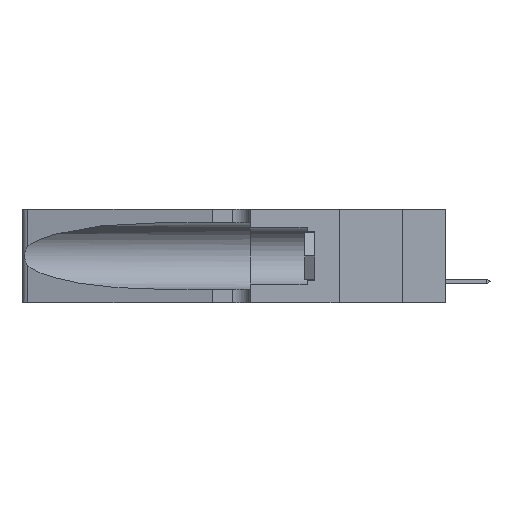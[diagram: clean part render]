
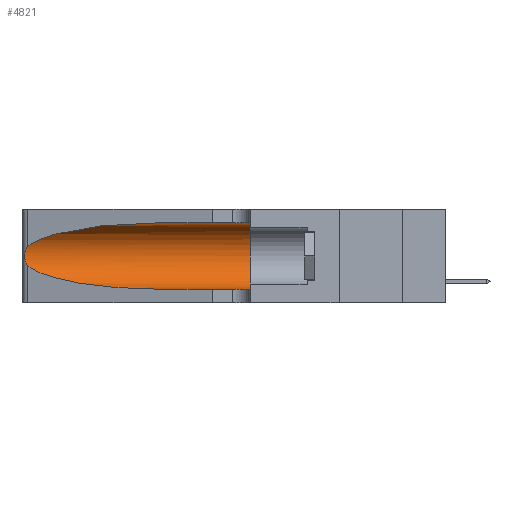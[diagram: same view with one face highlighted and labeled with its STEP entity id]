
A CAD part, left-side view. The second image highlights one B-rep face of the part: STEP entity #4821.
In plain terms, the highlighted cylindrical face has radius 3.308 mm (diameter 6.617 mm), a partial arc.
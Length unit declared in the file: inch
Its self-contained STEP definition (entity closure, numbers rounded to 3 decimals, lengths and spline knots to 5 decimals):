
#594 = B_SPLINE_CURVE_WITH_KNOTS ( 'NONE', 3,
 ( #18138, #36412, #43716, #26336, #4573, #8216, #18551, #36834, #26012, #4256, #18857, #44283, #20702, #31666 ),
 .UNSPECIFIED., .F., .F.,
 ( 4, 2, 2, 2, 2, 2, 4 ),
 ( 0., 0.00027, 0.00053, 0.00107, 0.0016, 0.00187, 0.00214 ),
 .UNSPECIFIED. ) ;
#1553 = DIRECTION ( 'NONE',  ( 0., -1., 0. ) ) ;
#2126 = EDGE_CURVE ( 'NONE', #46889, #8307, #594, .T. ) ;
#2876 = ORIENTED_EDGE ( 'NONE', *, *, #18980, .F. ) ;
#3038 = ORIENTED_EDGE ( 'NONE', *, *, #10313, .T. ) ;
#4256 = CARTESIAN_POINT ( 'NONE',  ( 0.25856, 1.23593, 0.16098 ) ) ;
#4573 = CARTESIAN_POINT ( 'NONE',  ( 0.25854, 1.2359, 0.20912 ) ) ;
#4821 = ADVANCED_FACE ( 'NONE', ( #39656 ), #5519, .F. ) ;
#4877 = VERTEX_POINT ( 'NONE', #45005 ) ;
#5519 = CYLINDRICAL_SURFACE ( 'NONE', #36890, 0.13025 ) ;
#7136 = CARTESIAN_POINT ( 'NONE',  ( 0.25487, 1.22718, 0.22369 ) ) ;
#8213 = CARTESIAN_POINT ( 'NONE',  ( 0.25487, 1.22718, 0.14631 ) ) ;
#8216 = CARTESIAN_POINT ( 'NONE',  ( 0.26018, 1.23835, 0.19895 ) ) ;
#8307 = VERTEX_POINT ( 'NONE', #28992 ) ;
#10313 = EDGE_CURVE ( 'NONE', #4877, #46889, #41458, .T. ) ;
#12385 = AXIS2_PLACEMENT_3D ( 'NONE', #45406, #28960, #24986 ) ;
#12713 = ORIENTED_EDGE ( 'NONE', *, *, #33773, .T. ) ;
#13643 = CARTESIAN_POINT ( 'NONE',  ( 0.1305, 0.35, 0.31525 ) ) ;
#15865 = CARTESIAN_POINT ( 'NONE',  ( 0.1305, 0.72297, 0.05475 ) ) ;
#16287 = DIRECTION ( 'NONE',  ( 0., -1., 0. ) ) ;
#17482 = CARTESIAN_POINT ( 'NONE',  ( 0.1305, 0.72297, 0.31525 ) ) ;
#17823 = VECTOR ( 'NONE', #1553, 39.37008 ) ;
#17933 = EDGE_CURVE ( 'NONE', #8307, #45367, #33846, .T. ) ;
#18040 = VERTEX_POINT ( 'NONE', #13643 ) ;
#18138 = CARTESIAN_POINT ( 'NONE',  ( 0.25487, 1.22718, 0.22369 ) ) ;
#18551 = CARTESIAN_POINT ( 'NONE',  ( 0.26075, 1.23896, 0.19203 ) ) ;
#18857 = CARTESIAN_POINT ( 'NONE',  ( 0.25789, 1.23486, 0.15765 ) ) ;
#18980 = EDGE_CURVE ( 'NONE', #18040, #36541, #40289, .T. ) ;
#20702 = CARTESIAN_POINT ( 'NONE',  ( 0.25555, 1.22993, 0.14849 ) ) ;
#20832 = EDGE_LOOP ( 'NONE', ( #3038, #37501, #43356, #12713, #2876, #32593 ) ) ;
#24986 = DIRECTION ( 'NONE',  ( 0., 0., 1. ) ) ;
#25980 = CARTESIAN_POINT ( 'NONE',  ( 0.1305, 1.61858, 0.05475 ) ) ;
#26012 = CARTESIAN_POINT ( 'NONE',  ( 0.26017, 1.23833, 0.17102 ) ) ;
#26336 = CARTESIAN_POINT ( 'NONE',  ( 0.25787, 1.23484, 0.2124 ) ) ;
#26826 = CARTESIAN_POINT ( 'NONE',  ( 0.18966, 0.96281, 0.31525 ) ) ;
#27161 = LINE ( 'NONE', #25980, #31167 ) ;
#28960 = DIRECTION ( 'NONE',  ( 0., 1., 0. ) ) ;
#28992 = CARTESIAN_POINT ( 'NONE',  ( 0.25487, 1.22718, 0.14631 ) ) ;
#30650 = CARTESIAN_POINT ( 'NONE',  ( 0.1305, 1.61858, 0.31525 ) ) ;
#31167 = VECTOR ( 'NONE', #37270, 39.37008 ) ;
#31666 = CARTESIAN_POINT ( 'NONE',  ( 0.25487, 1.22718, 0.14631 ) ) ;
#31929 = CARTESIAN_POINT ( 'NONE',  ( 0.1305, 0.72297, 0.05475 ) ) ;
#32593 = ORIENTED_EDGE ( 'NONE', *, *, #39405, .F. ) ;
#33497 = CARTESIAN_POINT ( 'NONE',  ( 0.18966, 0.96281, 0.05475 ) ) ;
#33773 = EDGE_CURVE ( 'NONE', #45367, #36541, #27161, .T. ) ;
#33846 =( BOUNDED_CURVE ( )  B_SPLINE_CURVE ( 3, ( #8213, #44763, #33497, #15865 ),
 .UNSPECIFIED., .F., .F. ) 
 B_SPLINE_CURVE_WITH_KNOTS ( ( 4, 4 ),
 ( 3.44316, 4.71239 ),
 .UNSPECIFIED. ) 
 CURVE ( )  GEOMETRIC_REPRESENTATION_ITEM ( )  RATIONAL_B_SPLINE_CURVE ( ( 1., 0.87, 0.87, 1. ) ) 
 REPRESENTATION_ITEM ( '' )  );
#34020 = CARTESIAN_POINT ( 'NONE',  ( 0.25487, 1.22718, 0.22369 ) ) ;
#34410 = CARTESIAN_POINT ( 'NONE',  ( 0.1305, 1.61858, 0.185 ) ) ;
#36390 = CARTESIAN_POINT ( 'NONE',  ( 0.1305, 0.35, 0.05475 ) ) ;
#36412 = CARTESIAN_POINT ( 'NONE',  ( 0.25555, 1.22994, 0.2215 ) ) ;
#36541 = VERTEX_POINT ( 'NONE', #36390 ) ;
#36834 = CARTESIAN_POINT ( 'NONE',  ( 0.26075, 1.23896, 0.178 ) ) ;
#36890 = AXIS2_PLACEMENT_3D ( 'NONE', #34410, #16287, #37906 ) ;
#37270 = DIRECTION ( 'NONE',  ( 0., -1., 0. ) ) ;
#37501 = ORIENTED_EDGE ( 'NONE', *, *, #2126, .T. ) ;
#37906 = DIRECTION ( 'NONE',  ( 0., 0., -1. ) ) ;
#39405 = EDGE_CURVE ( 'NONE', #4877, #18040, #45630, .T. ) ;
#39656 = FACE_OUTER_BOUND ( 'NONE', #20832, .T. ) ;
#39711 = CARTESIAN_POINT ( 'NONE',  ( 0.2373, 1.15595, 0.28018 ) ) ;
#40289 = CIRCLE ( 'NONE', #12385, 0.13025 ) ;
#41458 =( BOUNDED_CURVE ( )  B_SPLINE_CURVE ( 3, ( #17482, #26826, #39711, #7136 ),
 .UNSPECIFIED., .F., .F. ) 
 B_SPLINE_CURVE_WITH_KNOTS ( ( 4, 4 ),
 ( 1.5708, 2.84003 ),
 .UNSPECIFIED. ) 
 CURVE ( )  GEOMETRIC_REPRESENTATION_ITEM ( )  RATIONAL_B_SPLINE_CURVE ( ( 1., 0.87, 0.87, 1. ) ) 
 REPRESENTATION_ITEM ( '' )  );
#43356 = ORIENTED_EDGE ( 'NONE', *, *, #17933, .T. ) ;
#43716 = CARTESIAN_POINT ( 'NONE',  ( 0.25639, 1.23184, 0.21858 ) ) ;
#44283 = CARTESIAN_POINT ( 'NONE',  ( 0.25639, 1.23186, 0.15144 ) ) ;
#44763 = CARTESIAN_POINT ( 'NONE',  ( 0.2373, 1.15595, 0.08982 ) ) ;
#45005 = CARTESIAN_POINT ( 'NONE',  ( 0.1305, 0.72297, 0.31525 ) ) ;
#45367 = VERTEX_POINT ( 'NONE', #31929 ) ;
#45406 = CARTESIAN_POINT ( 'NONE',  ( 0.1305, 0.35, 0.185 ) ) ;
#45630 = LINE ( 'NONE', #30650, #17823 ) ;
#46889 = VERTEX_POINT ( 'NONE', #34020 ) ;
